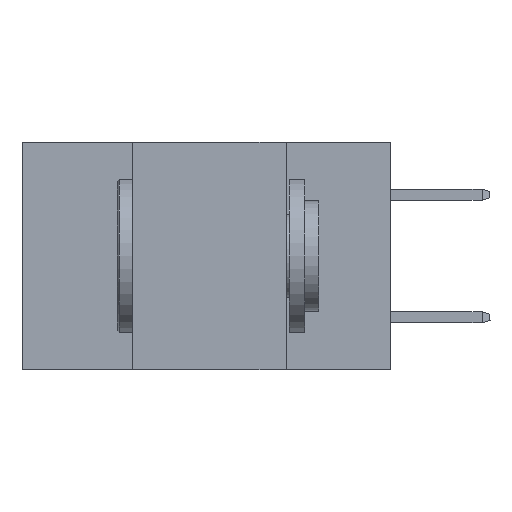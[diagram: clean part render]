
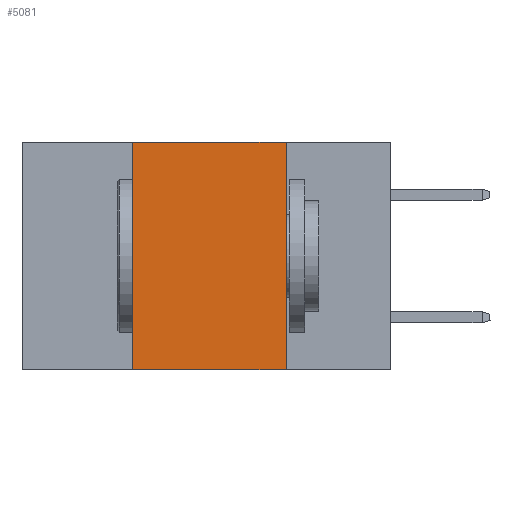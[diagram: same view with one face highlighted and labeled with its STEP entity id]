
A CAD part, left-side view. The second image highlights one B-rep face of the part: STEP entity #5081.
In plain terms, the highlighted planar face has unit normal (-1, 0, 0).
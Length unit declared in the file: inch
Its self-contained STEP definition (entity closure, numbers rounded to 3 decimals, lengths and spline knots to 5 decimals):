
#220 = DIRECTION ( 'NONE',  ( 0., -1., 0. ) ) ;
#1956 = PLANE ( 'NONE',  #15719 ) ;
#3787 = VECTOR ( 'NONE', #21650, 39.37008 ) ;
#5081 = ADVANCED_FACE ( 'NONE', ( #14365 ), #1956, .F. ) ;
#5757 = CARTESIAN_POINT ( 'NONE',  ( 0., 0.6, 0. ) ) ;
#6017 = VECTOR ( 'NONE', #20273, 39.37008 ) ;
#8381 = EDGE_CURVE ( 'NONE', #21481, #40866, #18211, .T. ) ;
#8922 = VECTOR ( 'NONE', #220, 39.37008 ) ;
#8995 = CARTESIAN_POINT ( 'NONE',  ( 0., 0.6, 0. ) ) ;
#9291 = ORIENTED_EDGE ( 'NONE', *, *, #38165, .F. ) ;
#9779 = ORIENTED_EDGE ( 'NONE', *, *, #20417, .F. ) ;
#11207 = CARTESIAN_POINT ( 'NONE',  ( 0., 0.17, -0.37 ) ) ;
#14365 = FACE_OUTER_BOUND ( 'NONE', #17074, .T. ) ;
#15719 = AXIS2_PLACEMENT_3D ( 'NONE', #8995, #28598, #35279 ) ;
#17074 = EDGE_LOOP ( 'NONE', ( #9779, #30312, #9291, #41854 ) ) ;
#18211 = LINE ( 'NONE', #5757, #3787 ) ;
#20273 = DIRECTION ( 'NONE',  ( 0., 0., -1. ) ) ;
#20417 = EDGE_CURVE ( 'NONE', #40866, #37114, #26745, .T. ) ;
#21481 = VERTEX_POINT ( 'NONE', #36893 ) ;
#21650 = DIRECTION ( 'NONE',  ( 0., -1., 0. ) ) ;
#26638 = EDGE_CURVE ( 'NONE', #31584, #37114, #30222, .T. ) ;
#26745 = LINE ( 'NONE', #40218, #6017 ) ;
#28598 = DIRECTION ( 'NONE',  ( 1., 0., 0. ) ) ;
#29125 = DIRECTION ( 'NONE',  ( 0., 0., 1. ) ) ;
#30176 = VECTOR ( 'NONE', #29125, 39.37008 ) ;
#30212 = CARTESIAN_POINT ( 'NONE',  ( 0., 0.42, -0.37 ) ) ;
#30222 = LINE ( 'NONE', #36908, #8922 ) ;
#30312 = ORIENTED_EDGE ( 'NONE', *, *, #8381, .F. ) ;
#30634 = CARTESIAN_POINT ( 'NONE',  ( 0., 0.17, 0. ) ) ;
#31584 = VERTEX_POINT ( 'NONE', #30212 ) ;
#34343 = LINE ( 'NONE', #39740, #30176 ) ;
#35279 = DIRECTION ( 'NONE',  ( 0., 0., -1. ) ) ;
#36893 = CARTESIAN_POINT ( 'NONE',  ( 0., 0.42, 0. ) ) ;
#36908 = CARTESIAN_POINT ( 'NONE',  ( 0., 0.6, -0.37 ) ) ;
#37114 = VERTEX_POINT ( 'NONE', #11207 ) ;
#38165 = EDGE_CURVE ( 'NONE', #31584, #21481, #34343, .T. ) ;
#39740 = CARTESIAN_POINT ( 'NONE',  ( 0., 0.42, 0. ) ) ;
#40218 = CARTESIAN_POINT ( 'NONE',  ( 0., 0.17, 0. ) ) ;
#40866 = VERTEX_POINT ( 'NONE', #30634 ) ;
#41854 = ORIENTED_EDGE ( 'NONE', *, *, #26638, .T. ) ;
